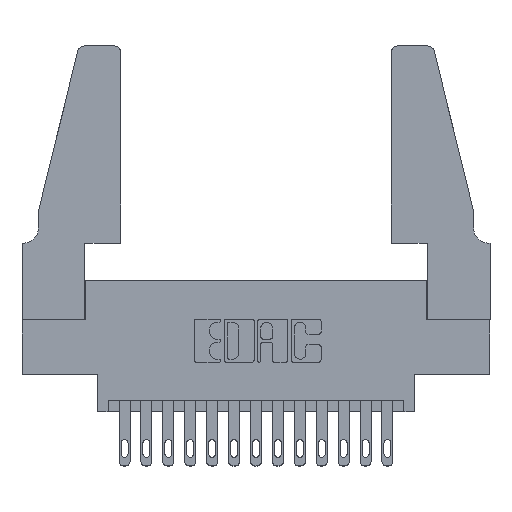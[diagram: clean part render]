
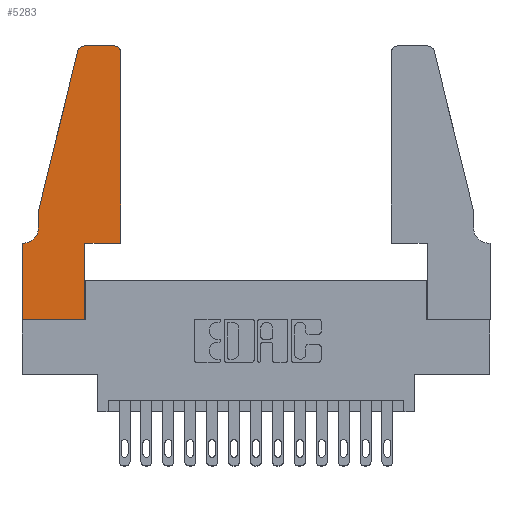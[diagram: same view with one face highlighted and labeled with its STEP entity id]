
A CAD part, top view. The second image highlights one B-rep face of the part: STEP entity #5283.
In plain terms, the highlighted planar face has unit normal (0, 0, 1).
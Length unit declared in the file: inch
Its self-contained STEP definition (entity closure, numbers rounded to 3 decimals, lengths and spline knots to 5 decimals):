
#433 = VECTOR ( 'NONE', #1632, 39.37008 ) ;
#656 = VERTEX_POINT ( 'NONE', #6013 ) ;
#731 = EDGE_CURVE ( 'NONE', #12879, #4181, #11672, .T. ) ;
#804 = VERTEX_POINT ( 'NONE', #3964 ) ;
#927 = DIRECTION ( 'NONE',  ( 0., 0., 1. ) ) ;
#995 = DIRECTION ( 'NONE',  ( 0., 0., 1. ) ) ;
#1024 = CARTESIAN_POINT ( 'NONE',  ( 0.2865, 0.35, 0.37 ) ) ;
#1083 = DIRECTION ( 'NONE',  ( 0., 1., 0. ) ) ;
#1205 = FACE_OUTER_BOUND ( 'NONE', #9120, .T. ) ;
#1207 = EDGE_CURVE ( 'NONE', #13016, #15379, #14364, .T. ) ;
#1583 = CARTESIAN_POINT ( 'NONE',  ( 0.2605, 1.25, 0.37 ) ) ;
#1630 = DIRECTION ( 'NONE',  ( 0., -1., 0. ) ) ;
#1632 = DIRECTION ( 'NONE',  ( 1., 0., 0. ) ) ;
#1806 = EDGE_CURVE ( 'NONE', #15379, #7176, #13747, .T. ) ;
#1928 = DIRECTION ( 'NONE',  ( 0., -1., 0. ) ) ;
#1950 = CARTESIAN_POINT ( 'NONE',  ( 0.4205, 1.25, 0.37 ) ) ;
#2308 = CARTESIAN_POINT ( 'NONE',  ( 0., 0.35, 0.37 ) ) ;
#2383 = VERTEX_POINT ( 'NONE', #12195 ) ;
#2400 = VECTOR ( 'NONE', #11296, 39.37008 ) ;
#2441 = ORIENTED_EDGE ( 'NONE', *, *, #15396, .T. ) ;
#2766 = CARTESIAN_POINT ( 'NONE',  ( 0., 0.35, 0.37 ) ) ;
#2929 = CARTESIAN_POINT ( 'NONE',  ( 0.0755, 0.5, 0.37 ) ) ;
#3215 = VERTEX_POINT ( 'NONE', #14345 ) ;
#3265 = CIRCLE ( 'NONE', #16061, 0.03 ) ;
#3511 = DIRECTION ( 'NONE',  ( 1., 0., 0. ) ) ;
#3770 = VECTOR ( 'NONE', #1630, 39.37008 ) ;
#3816 = VECTOR ( 'NONE', #11570, 39.37008 ) ;
#3964 = CARTESIAN_POINT ( 'NONE',  ( 0., 0., 0.37 ) ) ;
#4134 = ORIENTED_EDGE ( 'NONE', *, *, #6227, .T. ) ;
#4181 = VERTEX_POINT ( 'NONE', #11544 ) ;
#4259 = CARTESIAN_POINT ( 'NONE',  ( 0., 0., 0.37 ) ) ;
#4260 = CARTESIAN_POINT ( 'NONE',  ( 0.2865, 0., 0.37 ) ) ;
#4554 = LINE ( 'NONE', #4259, #3770 ) ;
#5020 = CARTESIAN_POINT ( 'NONE',  ( 0., 0., 0.37 ) ) ;
#5124 = EDGE_CURVE ( 'NONE', #2383, #3215, #13843, .T. ) ;
#5283 = ADVANCED_FACE ( 'NONE', ( #1205 ), #15502, .T. ) ;
#5357 = EDGE_CURVE ( 'NONE', #656, #8690, #13464, .T. ) ;
#5588 = EDGE_CURVE ( 'NONE', #804, #12879, #14432, .T. ) ;
#5593 = ORIENTED_EDGE ( 'NONE', *, *, #12671, .T. ) ;
#5642 = VECTOR ( 'NONE', #1928, 39.37008 ) ;
#5676 = VERTEX_POINT ( 'NONE', #10572 ) ;
#5983 = CARTESIAN_POINT ( 'NONE',  ( 0.4205, 1.22, 0.37 ) ) ;
#6013 = CARTESIAN_POINT ( 'NONE',  ( 0.0055, 0.35, 0.37 ) ) ;
#6210 = CARTESIAN_POINT ( 'NONE',  ( 0.4505, 0.35, 0.37 ) ) ;
#6227 = EDGE_CURVE ( 'NONE', #8690, #804, #4554, .T. ) ;
#6292 = DIRECTION ( 'NONE',  ( 0., 0., 1. ) ) ;
#6394 = DIRECTION ( 'NONE',  ( -1., 0., 0. ) ) ;
#6666 = AXIS2_PLACEMENT_3D ( 'NONE', #11187, #12669, #6394 ) ;
#6789 = DIRECTION ( 'NONE',  ( -1., 0., 0. ) ) ;
#6883 = ORIENTED_EDGE ( 'NONE', *, *, #5588, .T. ) ;
#7093 = DIRECTION ( 'NONE',  ( 1., 0., 0. ) ) ;
#7176 = VERTEX_POINT ( 'NONE', #1950 ) ;
#7550 = VECTOR ( 'NONE', #1083, 39.37008 ) ;
#7572 = DIRECTION ( 'NONE',  ( 1., 0., 0. ) ) ;
#8282 = CARTESIAN_POINT ( 'NONE',  ( 0.0755, 0.35, 0.37 ) ) ;
#8690 = VERTEX_POINT ( 'NONE', #2308 ) ;
#8832 = ORIENTED_EDGE ( 'NONE', *, *, #731, .T. ) ;
#8979 = VERTEX_POINT ( 'NONE', #11596 ) ;
#9120 = EDGE_LOOP ( 'NONE', ( #13369, #10405, #9557, #10746, #2441, #9392, #4134, #6883, #8832, #5593, #15947, #14602 ) ) ;
#9309 = VECTOR ( 'NONE', #6789, 39.37008 ) ;
#9392 = ORIENTED_EDGE ( 'NONE', *, *, #5357, .T. ) ;
#9557 = ORIENTED_EDGE ( 'NONE', *, *, #5124, .T. ) ;
#9972 = DIRECTION ( 'NONE',  ( 0., 1., 0. ) ) ;
#10084 = VECTOR ( 'NONE', #11445, 39.37008 ) ;
#10405 = ORIENTED_EDGE ( 'NONE', *, *, #11846, .T. ) ;
#10572 = CARTESIAN_POINT ( 'NONE',  ( 0.0755, 0.42, 0.37 ) ) ;
#10746 = ORIENTED_EDGE ( 'NONE', *, *, #15682, .T. ) ;
#11187 = CARTESIAN_POINT ( 'NONE',  ( 0.0055, 0.42, 0.37 ) ) ;
#11290 = LINE ( 'NONE', #13123, #433 ) ;
#11296 = DIRECTION ( 'NONE',  ( -0.239, -0.971, 0. ) ) ;
#11445 = DIRECTION ( 'NONE',  ( 1., 0., 0. ) ) ;
#11544 = CARTESIAN_POINT ( 'NONE',  ( 0.2865, 0.35, 0.37 ) ) ;
#11570 = DIRECTION ( 'NONE',  ( -1., 0., 0. ) ) ;
#11596 = CARTESIAN_POINT ( 'NONE',  ( 0.284, 1.25, 0.37 ) ) ;
#11672 = LINE ( 'NONE', #1024, #7550 ) ;
#11846 = EDGE_CURVE ( 'NONE', #8979, #2383, #3265, .T. ) ;
#12095 = LINE ( 'NONE', #1583, #3816 ) ;
#12195 = CARTESIAN_POINT ( 'NONE',  ( 0.25487, 1.22718, 0.37 ) ) ;
#12304 = CARTESIAN_POINT ( 'NONE',  ( 0.284, 1.22, 0.37 ) ) ;
#12607 = EDGE_CURVE ( 'NONE', #7176, #8979, #12095, .T. ) ;
#12669 = DIRECTION ( 'NONE',  ( 0., 0., -1. ) ) ;
#12671 = EDGE_CURVE ( 'NONE', #4181, #13016, #11290, .T. ) ;
#12879 = VERTEX_POINT ( 'NONE', #4260 ) ;
#13016 = VERTEX_POINT ( 'NONE', #14661 ) ;
#13123 = CARTESIAN_POINT ( 'NONE',  ( 0.4505, 0.35, 0.37 ) ) ;
#13150 = CIRCLE ( 'NONE', #6666, 0.07 ) ;
#13369 = ORIENTED_EDGE ( 'NONE', *, *, #12607, .T. ) ;
#13464 = LINE ( 'NONE', #8282, #9309 ) ;
#13518 = AXIS2_PLACEMENT_3D ( 'NONE', #5983, #995, #7093 ) ;
#13665 = AXIS2_PLACEMENT_3D ( 'NONE', #2766, #6292, #7572 ) ;
#13747 = CIRCLE ( 'NONE', #13518, 0.03 ) ;
#13762 = VECTOR ( 'NONE', #9972, 39.37008 ) ;
#13843 = LINE ( 'NONE', #16226, #2400 ) ;
#14323 = LINE ( 'NONE', #2929, #5642 ) ;
#14345 = CARTESIAN_POINT ( 'NONE',  ( 0.0755, 0.5, 0.37 ) ) ;
#14364 = LINE ( 'NONE', #6210, #13762 ) ;
#14432 = LINE ( 'NONE', #5020, #10084 ) ;
#14602 = ORIENTED_EDGE ( 'NONE', *, *, #1806, .T. ) ;
#14661 = CARTESIAN_POINT ( 'NONE',  ( 0.4505, 0.35, 0.37 ) ) ;
#14718 = CARTESIAN_POINT ( 'NONE',  ( 0.4505, 1.22, 0.37 ) ) ;
#15379 = VERTEX_POINT ( 'NONE', #14718 ) ;
#15396 = EDGE_CURVE ( 'NONE', #5676, #656, #13150, .T. ) ;
#15502 = PLANE ( 'NONE',  #13665 ) ;
#15682 = EDGE_CURVE ( 'NONE', #3215, #5676, #14323, .T. ) ;
#15947 = ORIENTED_EDGE ( 'NONE', *, *, #1207, .T. ) ;
#16061 = AXIS2_PLACEMENT_3D ( 'NONE', #12304, #927, #3511 ) ;
#16226 = CARTESIAN_POINT ( 'NONE',  ( 0.0755, 0.5, 0.37 ) ) ;
